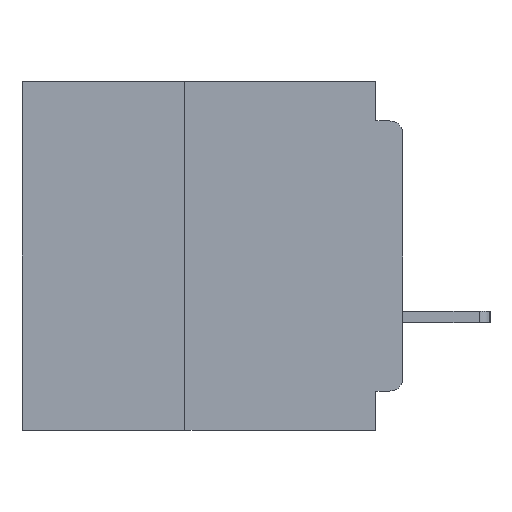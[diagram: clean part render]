
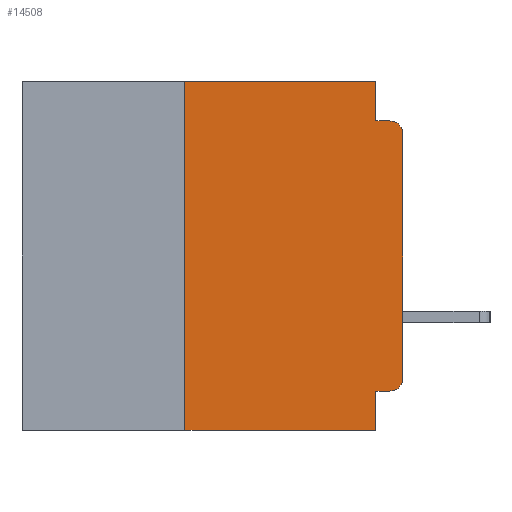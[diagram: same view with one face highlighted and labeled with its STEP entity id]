
A CAD part, left-side view. The second image highlights one B-rep face of the part: STEP entity #14508.
In plain terms, the highlighted planar face has unit normal (-1, 0, 0).
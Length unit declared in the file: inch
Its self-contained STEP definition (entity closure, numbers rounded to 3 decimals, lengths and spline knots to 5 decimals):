
#807 = LINE ( 'NONE', #15510, #8004 ) ;
#937 = DIRECTION ( 'NONE',  ( 0., 0., -1. ) ) ;
#1207 = VERTEX_POINT ( 'NONE', #31090 ) ;
#2018 = DIRECTION ( 'NONE',  ( -1., 0., 0. ) ) ;
#3202 = CARTESIAN_POINT ( 'NONE',  ( 0., 0.437, -0.4 ) ) ;
#4112 = VERTEX_POINT ( 'NONE', #38319 ) ;
#6256 = VERTEX_POINT ( 'NONE', #25473 ) ;
#6343 = VECTOR ( 'NONE', #10970, 39.37008 ) ;
#8004 = VECTOR ( 'NONE', #24529, 39.37008 ) ;
#8259 = CARTESIAN_POINT ( 'NONE',  ( 0., 0., -0.34 ) ) ;
#9982 = CARTESIAN_POINT ( 'NONE',  ( 0., 0.031, -0.4 ) ) ;
#10321 = CIRCLE ( 'NONE', #24312, 0.015 ) ;
#10970 = DIRECTION ( 'NONE',  ( 0., 0., 1. ) ) ;
#11073 = EDGE_LOOP ( 'NONE', ( #35864, #30890, #12116, #34209, #16765, #13358, #33072, #33128, #31423, #36283 ) ) ;
#11744 = AXIS2_PLACEMENT_3D ( 'NONE', #13824, #34931, #16840 ) ;
#12116 = ORIENTED_EDGE ( 'NONE', *, *, #28642, .F. ) ;
#12729 = CARTESIAN_POINT ( 'NONE',  ( 0., 0.031, -0.4 ) ) ;
#13358 = ORIENTED_EDGE ( 'NONE', *, *, #20521, .F. ) ;
#13465 = VECTOR ( 'NONE', #937, 39.37008 ) ;
#13591 = FACE_OUTER_BOUND ( 'NONE', #11073, .T. ) ;
#13824 = CARTESIAN_POINT ( 'NONE',  ( 0., 0.015, -0.06 ) ) ;
#13957 = CARTESIAN_POINT ( 'NONE',  ( 0., 0.437, 0. ) ) ;
#14490 = EDGE_CURVE ( 'NONE', #4112, #20742, #14556, .T. ) ;
#14508 = ADVANCED_FACE ( 'NONE', ( #13591 ), #31995, .F. ) ;
#14556 = CIRCLE ( 'NONE', #11744, 0.015 ) ;
#14987 = CARTESIAN_POINT ( 'NONE',  ( 0., 0., -0.045 ) ) ;
#15355 = LINE ( 'NONE', #27902, #22372 ) ;
#15359 = DIRECTION ( 'NONE',  ( 0., -1., 0. ) ) ;
#15510 = CARTESIAN_POINT ( 'NONE',  ( 0., 0.437, 0. ) ) ;
#16259 = CARTESIAN_POINT ( 'NONE',  ( 0., 0.25, -0.4 ) ) ;
#16513 = CARTESIAN_POINT ( 'NONE',  ( 0., 0.25, -0.4 ) ) ;
#16765 = ORIENTED_EDGE ( 'NONE', *, *, #21537, .F. ) ;
#16840 = DIRECTION ( 'NONE',  ( 0., 0., -1. ) ) ;
#16976 = DIRECTION ( 'NONE',  ( 1., 0., 0. ) ) ;
#17308 = CARTESIAN_POINT ( 'NONE',  ( 0., 0.031, -0.045 ) ) ;
#19639 = VECTOR ( 'NONE', #24025, 39.37008 ) ;
#20047 = LINE ( 'NONE', #3202, #27130 ) ;
#20097 = CARTESIAN_POINT ( 'NONE',  ( 0., 0.015, -0.34 ) ) ;
#20521 = EDGE_CURVE ( 'NONE', #35660, #22473, #22618, .T. ) ;
#20742 = VERTEX_POINT ( 'NONE', #26613 ) ;
#21436 = LINE ( 'NONE', #9982, #13465 ) ;
#21537 = EDGE_CURVE ( 'NONE', #22473, #1207, #807, .T. ) ;
#21683 = VECTOR ( 'NONE', #22375, 39.37008 ) ;
#21810 = AXIS2_PLACEMENT_3D ( 'NONE', #13957, #16976, #38056 ) ;
#21916 = VERTEX_POINT ( 'NONE', #17308 ) ;
#22306 = LINE ( 'NONE', #23038, #6343 ) ;
#22372 = VECTOR ( 'NONE', #33972, 39.37008 ) ;
#22375 = DIRECTION ( 'NONE',  ( 0., 0., 1. ) ) ;
#22473 = VERTEX_POINT ( 'NONE', #33146 ) ;
#22618 = LINE ( 'NONE', #16513, #21683 ) ;
#23038 = CARTESIAN_POINT ( 'NONE',  ( 0., 0., 0. ) ) ;
#23102 = DIRECTION ( 'NONE',  ( 0., 0., -1. ) ) ;
#23864 = VERTEX_POINT ( 'NONE', #12729 ) ;
#23886 = EDGE_CURVE ( 'NONE', #6256, #35318, #15355, .T. ) ;
#23902 = EDGE_CURVE ( 'NONE', #35318, #23864, #21436, .T. ) ;
#24025 = DIRECTION ( 'NONE',  ( 0., -1., 0. ) ) ;
#24312 = AXIS2_PLACEMENT_3D ( 'NONE', #20097, #2018, #23102 ) ;
#24529 = DIRECTION ( 'NONE',  ( 0., -1., 0. ) ) ;
#24770 = EDGE_CURVE ( 'NONE', #35270, #4112, #22306, .T. ) ;
#25473 = CARTESIAN_POINT ( 'NONE',  ( 0., 0.015, -0.355 ) ) ;
#26613 = CARTESIAN_POINT ( 'NONE',  ( 0., 0.015, -0.045 ) ) ;
#27017 = CARTESIAN_POINT ( 'NONE',  ( 0., 0.031, 0. ) ) ;
#27130 = VECTOR ( 'NONE', #15359, 39.37008 ) ;
#27474 = LINE ( 'NONE', #27017, #37380 ) ;
#27902 = CARTESIAN_POINT ( 'NONE',  ( 0., 0., -0.355 ) ) ;
#28642 = EDGE_CURVE ( 'NONE', #21916, #20742, #37587, .T. ) ;
#30069 = DIRECTION ( 'NONE',  ( 0., 0., -1. ) ) ;
#30890 = ORIENTED_EDGE ( 'NONE', *, *, #14490, .T. ) ;
#31090 = CARTESIAN_POINT ( 'NONE',  ( 0., 0.031, 0. ) ) ;
#31423 = ORIENTED_EDGE ( 'NONE', *, *, #23886, .F. ) ;
#31995 = PLANE ( 'NONE',  #21810 ) ;
#32469 = CARTESIAN_POINT ( 'NONE',  ( 0., 0.031, -0.355 ) ) ;
#33072 = ORIENTED_EDGE ( 'NONE', *, *, #38806, .T. ) ;
#33128 = ORIENTED_EDGE ( 'NONE', *, *, #23902, .F. ) ;
#33146 = CARTESIAN_POINT ( 'NONE',  ( 0., 0.25, 0. ) ) ;
#33377 = EDGE_CURVE ( 'NONE', #1207, #21916, #27474, .T. ) ;
#33972 = DIRECTION ( 'NONE',  ( 0., 1., 0. ) ) ;
#34209 = ORIENTED_EDGE ( 'NONE', *, *, #33377, .F. ) ;
#34931 = DIRECTION ( 'NONE',  ( -1., 0., 0. ) ) ;
#35270 = VERTEX_POINT ( 'NONE', #8259 ) ;
#35318 = VERTEX_POINT ( 'NONE', #32469 ) ;
#35660 = VERTEX_POINT ( 'NONE', #16259 ) ;
#35864 = ORIENTED_EDGE ( 'NONE', *, *, #24770, .T. ) ;
#36283 = ORIENTED_EDGE ( 'NONE', *, *, #36464, .T. ) ;
#36464 = EDGE_CURVE ( 'NONE', #6256, #35270, #10321, .T. ) ;
#37380 = VECTOR ( 'NONE', #30069, 39.37008 ) ;
#37587 = LINE ( 'NONE', #14987, #19639 ) ;
#38056 = DIRECTION ( 'NONE',  ( 0., 0., -1. ) ) ;
#38319 = CARTESIAN_POINT ( 'NONE',  ( 0., 0., -0.06 ) ) ;
#38806 = EDGE_CURVE ( 'NONE', #35660, #23864, #20047, .T. ) ;
